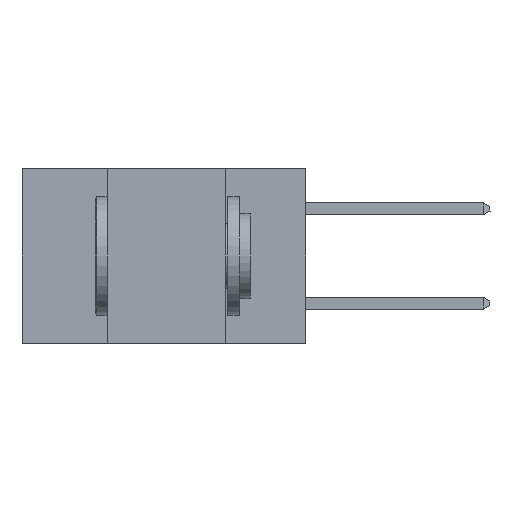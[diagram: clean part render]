
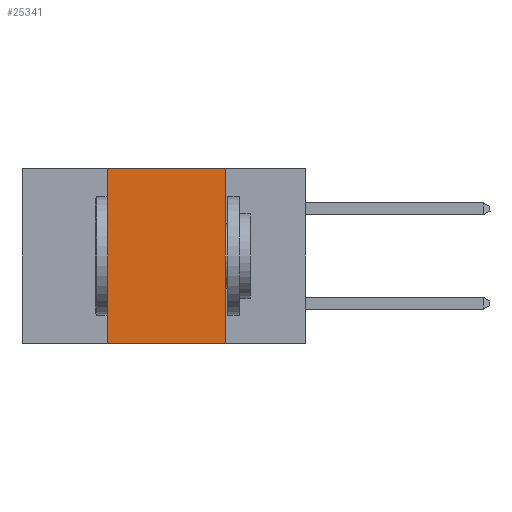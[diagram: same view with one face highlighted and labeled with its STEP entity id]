
A CAD part, left-side view. The second image highlights one B-rep face of the part: STEP entity #25341.
In plain terms, the highlighted planar face has unit normal (-1, 0, 0).
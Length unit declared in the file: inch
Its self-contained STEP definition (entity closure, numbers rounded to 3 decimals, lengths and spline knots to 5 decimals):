
#137 = DIRECTION ( 'NONE',  ( 1., 0., 0. ) ) ;
#1132 = ORIENTED_EDGE ( 'NONE', *, *, #12193, .F. ) ;
#3203 = CARTESIAN_POINT ( 'NONE',  ( 0., 0.6, -0.37 ) ) ;
#4031 = EDGE_CURVE ( 'NONE', #8377, #4976, #12427, .T. ) ;
#4622 = CARTESIAN_POINT ( 'NONE',  ( 0., 0.6, 0. ) ) ;
#4976 = VERTEX_POINT ( 'NONE', #17679 ) ;
#5252 = LINE ( 'NONE', #6426, #23102 ) ;
#6426 = CARTESIAN_POINT ( 'NONE',  ( 0., 0.17, 0. ) ) ;
#7190 = CARTESIAN_POINT ( 'NONE',  ( 0., 0.6, 0. ) ) ;
#8377 = VERTEX_POINT ( 'NONE', #19658 ) ;
#8410 = EDGE_CURVE ( 'NONE', #16699, #8377, #24888, .T. ) ;
#9244 = VERTEX_POINT ( 'NONE', #11012 ) ;
#10373 = DIRECTION ( 'NONE',  ( 0., 0., 1. ) ) ;
#10427 = ORIENTED_EDGE ( 'NONE', *, *, #13393, .T. ) ;
#11012 = CARTESIAN_POINT ( 'NONE',  ( 0., 0.17, -0.37 ) ) ;
#11261 = DIRECTION ( 'NONE',  ( 0., -1., 0. ) ) ;
#11673 = VECTOR ( 'NONE', #11261, 39.37008 ) ;
#12193 = EDGE_CURVE ( 'NONE', #4976, #9244, #5252, .T. ) ;
#12427 = LINE ( 'NONE', #4622, #11673 ) ;
#13393 = EDGE_CURVE ( 'NONE', #16699, #9244, #21537, .T. ) ;
#13711 = DIRECTION ( 'NONE',  ( 0., 0., -1. ) ) ;
#15440 = VECTOR ( 'NONE', #10373, 39.37008 ) ;
#15946 = FACE_OUTER_BOUND ( 'NONE', #24963, .T. ) ;
#16699 = VERTEX_POINT ( 'NONE', #29159 ) ;
#17679 = CARTESIAN_POINT ( 'NONE',  ( 0., 0.17, 0. ) ) ;
#18409 = PLANE ( 'NONE',  #22182 ) ;
#18792 = ORIENTED_EDGE ( 'NONE', *, *, #4031, .F. ) ;
#19513 = DIRECTION ( 'NONE',  ( 0., -1., 0. ) ) ;
#19658 = CARTESIAN_POINT ( 'NONE',  ( 0., 0.42, 0. ) ) ;
#20780 = ORIENTED_EDGE ( 'NONE', *, *, #8410, .F. ) ;
#21537 = LINE ( 'NONE', #3203, #24105 ) ;
#22182 = AXIS2_PLACEMENT_3D ( 'NONE', #7190, #137, #13711 ) ;
#22275 = CARTESIAN_POINT ( 'NONE',  ( 0., 0.42, 0. ) ) ;
#22711 = DIRECTION ( 'NONE',  ( 0., 0., -1. ) ) ;
#23102 = VECTOR ( 'NONE', #22711, 39.37008 ) ;
#24105 = VECTOR ( 'NONE', #19513, 39.37008 ) ;
#24888 = LINE ( 'NONE', #22275, #15440 ) ;
#24963 = EDGE_LOOP ( 'NONE', ( #1132, #18792, #20780, #10427 ) ) ;
#25341 = ADVANCED_FACE ( 'NONE', ( #15946 ), #18409, .F. ) ;
#29159 = CARTESIAN_POINT ( 'NONE',  ( 0., 0.42, -0.37 ) ) ;
